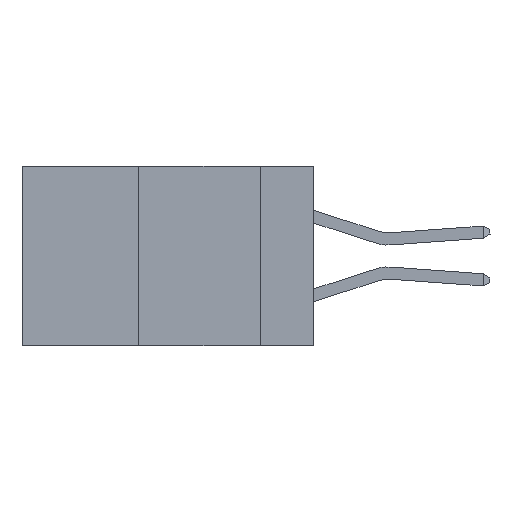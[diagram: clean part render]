
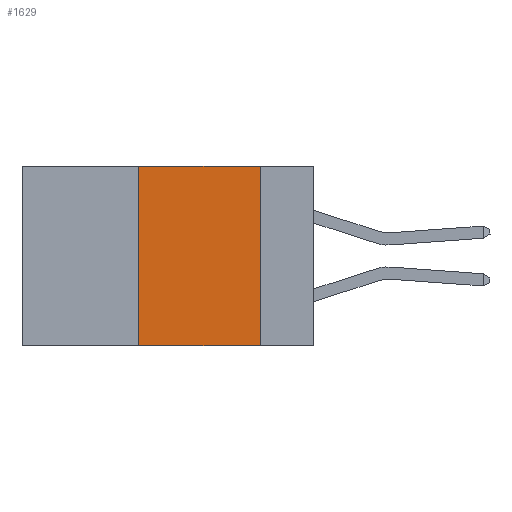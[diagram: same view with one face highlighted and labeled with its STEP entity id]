
A CAD part, left-side view. The second image highlights one B-rep face of the part: STEP entity #1629.
In plain terms, the highlighted planar face has unit normal (-1, 0, 0).
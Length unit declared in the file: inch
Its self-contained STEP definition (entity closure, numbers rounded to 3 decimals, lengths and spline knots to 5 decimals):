
#108 = DIRECTION ( 'NONE',  ( 0., 0., 1. ) ) ;
#661 = DIRECTION ( 'NONE',  ( 0., -1., 0. ) ) ;
#801 = ORIENTED_EDGE ( 'NONE', *, *, #24058, .F. ) ;
#1151 = FACE_OUTER_BOUND ( 'NONE', #27185, .T. ) ;
#1629 = ADVANCED_FACE ( 'NONE', ( #1151 ), #12158, .F. ) ;
#1978 = AXIS2_PLACEMENT_3D ( 'NONE', #33114, #36140, #18216 ) ;
#2208 = VECTOR ( 'NONE', #8235, 39.37008 ) ;
#2838 = LINE ( 'NONE', #6270, #33863 ) ;
#3171 = LINE ( 'NONE', #32257, #2208 ) ;
#6270 = CARTESIAN_POINT ( 'NONE',  ( 0., 0.6, -0.37 ) ) ;
#7934 = CARTESIAN_POINT ( 'NONE',  ( 0., 0.11, 0. ) ) ;
#7990 = VERTEX_POINT ( 'NONE', #19905 ) ;
#8235 = DIRECTION ( 'NONE',  ( 0., 0., -1. ) ) ;
#9464 = VECTOR ( 'NONE', #661, 39.37008 ) ;
#10612 = VERTEX_POINT ( 'NONE', #35146 ) ;
#12158 = PLANE ( 'NONE',  #1978 ) ;
#12483 = DIRECTION ( 'NONE',  ( 0., -1., 0. ) ) ;
#12742 = CARTESIAN_POINT ( 'NONE',  ( 0., 0.6, 0. ) ) ;
#13286 = VECTOR ( 'NONE', #108, 39.37008 ) ;
#13654 = EDGE_CURVE ( 'NONE', #23218, #10612, #2838, .T. ) ;
#18216 = DIRECTION ( 'NONE',  ( 0., 0., -1. ) ) ;
#18316 = ORIENTED_EDGE ( 'NONE', *, *, #27274, .F. ) ;
#18810 = ORIENTED_EDGE ( 'NONE', *, *, #31517, .F. ) ;
#19905 = CARTESIAN_POINT ( 'NONE',  ( 0., 0.36, 0. ) ) ;
#22220 = LINE ( 'NONE', #24146, #13286 ) ;
#23218 = VERTEX_POINT ( 'NONE', #32326 ) ;
#24058 = EDGE_CURVE ( 'NONE', #7990, #33818, #33379, .T. ) ;
#24146 = CARTESIAN_POINT ( 'NONE',  ( 0., 0.36, 0. ) ) ;
#25654 = ORIENTED_EDGE ( 'NONE', *, *, #13654, .T. ) ;
#27185 = EDGE_LOOP ( 'NONE', ( #18316, #801, #18810, #25654 ) ) ;
#27274 = EDGE_CURVE ( 'NONE', #33818, #10612, #3171, .T. ) ;
#31517 = EDGE_CURVE ( 'NONE', #23218, #7990, #22220, .T. ) ;
#32257 = CARTESIAN_POINT ( 'NONE',  ( 0., 0.11, 0. ) ) ;
#32326 = CARTESIAN_POINT ( 'NONE',  ( 0., 0.36, -0.37 ) ) ;
#33114 = CARTESIAN_POINT ( 'NONE',  ( 0., 0.6, 0. ) ) ;
#33379 = LINE ( 'NONE', #12742, #9464 ) ;
#33818 = VERTEX_POINT ( 'NONE', #7934 ) ;
#33863 = VECTOR ( 'NONE', #12483, 39.37008 ) ;
#35146 = CARTESIAN_POINT ( 'NONE',  ( 0., 0.11, -0.37 ) ) ;
#36140 = DIRECTION ( 'NONE',  ( 1., 0., 0. ) ) ;
